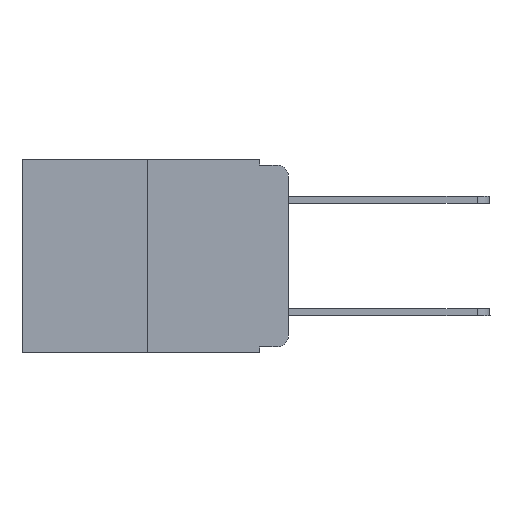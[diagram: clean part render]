
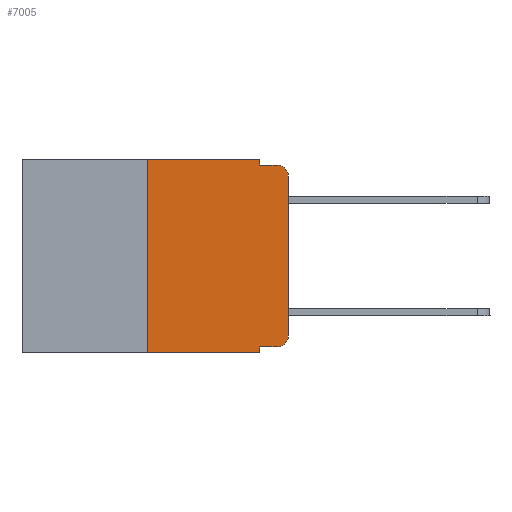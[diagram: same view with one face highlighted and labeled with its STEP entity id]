
A CAD part, left-side view. The second image highlights one B-rep face of the part: STEP entity #7005.
In plain terms, the highlighted planar face has unit normal (-1, 0, 0).
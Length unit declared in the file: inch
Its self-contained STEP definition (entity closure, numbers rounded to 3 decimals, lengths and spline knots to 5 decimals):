
#53 = LINE ( 'NONE', #12994, #10721 ) ;
#80 = DIRECTION ( 'NONE',  ( 0., -1., 0. ) ) ;
#274 = VECTOR ( 'NONE', #11190, 39.37008 ) ;
#456 = VERTEX_POINT ( 'NONE', #10164 ) ;
#563 = DIRECTION ( 'NONE',  ( 0., 0., -1. ) ) ;
#667 = VERTEX_POINT ( 'NONE', #3792 ) ;
#716 = EDGE_CURVE ( 'NONE', #456, #5541, #2664, .T. ) ;
#724 = ORIENTED_EDGE ( 'NONE', *, *, #2498, .T. ) ;
#838 = CARTESIAN_POINT ( 'NONE',  ( 0., 0.051, -0.01 ) ) ;
#839 = CARTESIAN_POINT ( 'NONE',  ( 0., 0.051, -0.343 ) ) ;
#957 = DIRECTION ( 'NONE',  ( 0., 0., -1. ) ) ;
#1342 = DIRECTION ( 'NONE',  ( -1., 0., 0. ) ) ;
#1364 = VERTEX_POINT ( 'NONE', #9450 ) ;
#1367 = CARTESIAN_POINT ( 'NONE',  ( 0., 0.051, -0.333 ) ) ;
#1472 = LINE ( 'NONE', #3913, #3338 ) ;
#1644 = VECTOR ( 'NONE', #80, 39.37008 ) ;
#1730 = VERTEX_POINT ( 'NONE', #1771 ) ;
#1771 = CARTESIAN_POINT ( 'NONE',  ( 0., 0.02, -0.01 ) ) ;
#2252 = EDGE_CURVE ( 'NONE', #5913, #1730, #12850, .T. ) ;
#2271 = VERTEX_POINT ( 'NONE', #9559 ) ;
#2452 = ORIENTED_EDGE ( 'NONE', *, *, #7198, .T. ) ;
#2498 = EDGE_CURVE ( 'NONE', #6936, #1364, #2505, .T. ) ;
#2505 = CIRCLE ( 'NONE', #6410, 0.02 ) ;
#2536 = FACE_OUTER_BOUND ( 'NONE', #8394, .T. ) ;
#2664 = LINE ( 'NONE', #6332, #7493 ) ;
#2670 = VECTOR ( 'NONE', #7086, 39.37008 ) ;
#2894 = EDGE_CURVE ( 'NONE', #2271, #7953, #12153, .T. ) ;
#2992 = LINE ( 'NONE', #4043, #274 ) ;
#3338 = VECTOR ( 'NONE', #9828, 39.37008 ) ;
#3792 = CARTESIAN_POINT ( 'NONE',  ( 0., 0.051, -0.333 ) ) ;
#3913 = CARTESIAN_POINT ( 'NONE',  ( 0., 0.051, 0. ) ) ;
#4041 = EDGE_CURVE ( 'NONE', #667, #6936, #9426, .T. ) ;
#4043 = CARTESIAN_POINT ( 'NONE',  ( 0., 0., 0. ) ) ;
#4533 = CARTESIAN_POINT ( 'NONE',  ( 0., 0.25, 0. ) ) ;
#4968 = EDGE_CURVE ( 'NONE', #667, #5541, #1472, .T. ) ;
#5451 = VECTOR ( 'NONE', #11228, 39.37008 ) ;
#5541 = VERTEX_POINT ( 'NONE', #839 ) ;
#5563 = ORIENTED_EDGE ( 'NONE', *, *, #716, .T. ) ;
#5821 = CARTESIAN_POINT ( 'NONE',  ( 0., 0.473, 0. ) ) ;
#5865 = CARTESIAN_POINT ( 'NONE',  ( 0., 0.051, 0. ) ) ;
#5913 = VERTEX_POINT ( 'NONE', #13360 ) ;
#5932 = DIRECTION ( 'NONE',  ( 0., 0., -1. ) ) ;
#6252 = AXIS2_PLACEMENT_3D ( 'NONE', #11845, #1342, #5932 ) ;
#6332 = CARTESIAN_POINT ( 'NONE',  ( 0., 0.473, -0.343 ) ) ;
#6410 = AXIS2_PLACEMENT_3D ( 'NONE', #12445, #13642, #957 ) ;
#6545 = CARTESIAN_POINT ( 'NONE',  ( 0., 0.473, 0. ) ) ;
#6882 = ORIENTED_EDGE ( 'NONE', *, *, #10999, .F. ) ;
#6936 = VERTEX_POINT ( 'NONE', #7334 ) ;
#6951 = LINE ( 'NONE', #11122, #14355 ) ;
#7005 = ADVANCED_FACE ( 'NONE', ( #2536 ), #11661, .F. ) ;
#7086 = DIRECTION ( 'NONE',  ( 0., 0., 1. ) ) ;
#7101 = DIRECTION ( 'NONE',  ( 0., -1., 0. ) ) ;
#7198 = EDGE_CURVE ( 'NONE', #1364, #5913, #2992, .T. ) ;
#7334 = CARTESIAN_POINT ( 'NONE',  ( 0., 0.02, -0.333 ) ) ;
#7470 = ORIENTED_EDGE ( 'NONE', *, *, #4968, .F. ) ;
#7493 = VECTOR ( 'NONE', #12236, 39.37008 ) ;
#7953 = VERTEX_POINT ( 'NONE', #5865 ) ;
#8394 = EDGE_LOOP ( 'NONE', ( #2452, #12610, #6882, #12163, #14122, #10098, #5563, #7470, #13947, #724 ) ) ;
#9071 = VERTEX_POINT ( 'NONE', #838 ) ;
#9426 = LINE ( 'NONE', #1367, #1644 ) ;
#9450 = CARTESIAN_POINT ( 'NONE',  ( 0., 0., -0.313 ) ) ;
#9559 = CARTESIAN_POINT ( 'NONE',  ( 0., 0.25, 0. ) ) ;
#9828 = DIRECTION ( 'NONE',  ( 0., 0., -1. ) ) ;
#10098 = ORIENTED_EDGE ( 'NONE', *, *, #12508, .F. ) ;
#10164 = CARTESIAN_POINT ( 'NONE',  ( 0., 0.25, -0.343 ) ) ;
#10446 = EDGE_CURVE ( 'NONE', #7953, #9071, #6951, .T. ) ;
#10721 = VECTOR ( 'NONE', #7101, 39.37008 ) ;
#10999 = EDGE_CURVE ( 'NONE', #9071, #1730, #53, .T. ) ;
#11122 = CARTESIAN_POINT ( 'NONE',  ( 0., 0.051, 0. ) ) ;
#11190 = DIRECTION ( 'NONE',  ( 0., 0., 1. ) ) ;
#11228 = DIRECTION ( 'NONE',  ( 0., -1., 0. ) ) ;
#11661 = PLANE ( 'NONE',  #14062 ) ;
#11845 = CARTESIAN_POINT ( 'NONE',  ( 0., 0.02, -0.03 ) ) ;
#11962 = DIRECTION ( 'NONE',  ( 1., 0., 0. ) ) ;
#12153 = LINE ( 'NONE', #6545, #5451 ) ;
#12163 = ORIENTED_EDGE ( 'NONE', *, *, #10446, .F. ) ;
#12236 = DIRECTION ( 'NONE',  ( 0., -1., 0. ) ) ;
#12445 = CARTESIAN_POINT ( 'NONE',  ( 0., 0.02, -0.313 ) ) ;
#12508 = EDGE_CURVE ( 'NONE', #456, #2271, #14110, .T. ) ;
#12610 = ORIENTED_EDGE ( 'NONE', *, *, #2252, .T. ) ;
#12850 = CIRCLE ( 'NONE', #6252, 0.02 ) ;
#12994 = CARTESIAN_POINT ( 'NONE',  ( 0., 0.051, -0.01 ) ) ;
#13360 = CARTESIAN_POINT ( 'NONE',  ( 0., 0., -0.03 ) ) ;
#13642 = DIRECTION ( 'NONE',  ( -1., 0., 0. ) ) ;
#13947 = ORIENTED_EDGE ( 'NONE', *, *, #4041, .T. ) ;
#14010 = DIRECTION ( 'NONE',  ( 0., 0., -1. ) ) ;
#14062 = AXIS2_PLACEMENT_3D ( 'NONE', #5821, #11962, #14010 ) ;
#14110 = LINE ( 'NONE', #4533, #2670 ) ;
#14122 = ORIENTED_EDGE ( 'NONE', *, *, #2894, .F. ) ;
#14355 = VECTOR ( 'NONE', #563, 39.37008 ) ;
